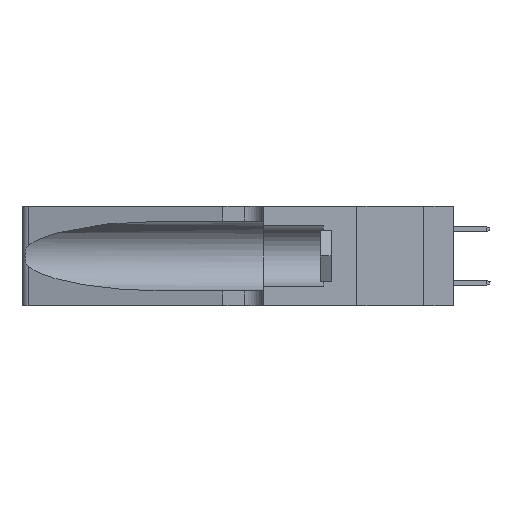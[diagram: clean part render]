
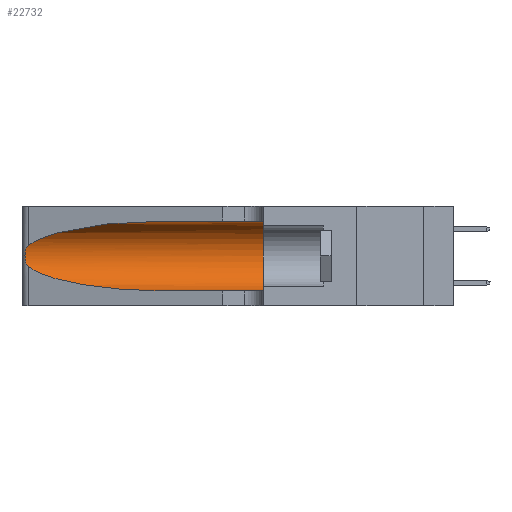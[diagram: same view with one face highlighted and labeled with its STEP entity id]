
A CAD part, left-side view. The second image highlights one B-rep face of the part: STEP entity #22732.
In plain terms, the highlighted cylindrical face has radius 3.308 mm (diameter 6.617 mm), a partial arc.
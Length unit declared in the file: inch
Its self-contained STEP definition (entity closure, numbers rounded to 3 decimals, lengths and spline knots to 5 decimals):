
#939 = VERTEX_POINT ( 'NONE', #15543 ) ;
#1526 = CARTESIAN_POINT ( 'NONE',  ( 0.2373, 1.15595, 0.08982 ) ) ;
#2543 = B_SPLINE_CURVE_WITH_KNOTS ( 'NONE', 3,
 ( #40751, #30170, #37373, #23429, #13076, #10136, #23860, #37588, #13746, #6750, #24303, #27682, #26802, #27464 ),
 .UNSPECIFIED., .F., .F.,
 ( 4, 2, 2, 2, 2, 2, 4 ),
 ( 0., 0.00027, 0.00053, 0.00107, 0.0016, 0.00187, 0.00214 ),
 .UNSPECIFIED. ) ;
#2754 = ORIENTED_EDGE ( 'NONE', *, *, #42380, .T. ) ;
#2977 = EDGE_LOOP ( 'NONE', ( #14669, #41446, #18980, #2754, #42474, #29948 ) ) ;
#4268 = CARTESIAN_POINT ( 'NONE',  ( 0.1305, 0.35, 0.31525 ) ) ;
#5178 = LINE ( 'NONE', #26124, #29187 ) ;
#5427 = CARTESIAN_POINT ( 'NONE',  ( 0.1305, 0.35, 0.185 ) ) ;
#6022 = DIRECTION ( 'NONE',  ( 0., 0., -1. ) ) ;
#6558 = EDGE_CURVE ( 'NONE', #7128, #14911, #5178, .T. ) ;
#6750 = CARTESIAN_POINT ( 'NONE',  ( 0.25856, 1.23593, 0.16098 ) ) ;
#7128 = VERTEX_POINT ( 'NONE', #16170 ) ;
#9047 = CARTESIAN_POINT ( 'NONE',  ( 0.1305, 1.61858, 0.05475 ) ) ;
#10136 = CARTESIAN_POINT ( 'NONE',  ( 0.26018, 1.23835, 0.19895 ) ) ;
#10517 = AXIS2_PLACEMENT_3D ( 'NONE', #29884, #30325, #6022 ) ;
#11136 = CARTESIAN_POINT ( 'NONE',  ( 0.25487, 1.22718, 0.22369 ) ) ;
#11793 = CARTESIAN_POINT ( 'NONE',  ( 0.18966, 0.96281, 0.31525 ) ) ;
#12193 = DIRECTION ( 'NONE',  ( 0., 1., 0. ) ) ;
#12660 = EDGE_CURVE ( 'NONE', #7128, #15549, #13015, .T. ) ;
#12906 = CIRCLE ( 'NONE', #36617, 0.13025 ) ;
#12931 = VECTOR ( 'NONE', #24326, 39.37008 ) ;
#13015 =( BOUNDED_CURVE ( )  B_SPLINE_CURVE ( 3, ( #35007, #11793, #15176, #11136 ),
 .UNSPECIFIED., .F., .F. ) 
 B_SPLINE_CURVE_WITH_KNOTS ( ( 4, 4 ),
 ( 1.5708, 2.84003 ),
 .UNSPECIFIED. ) 
 CURVE ( )  GEOMETRIC_REPRESENTATION_ITEM ( )  RATIONAL_B_SPLINE_CURVE ( ( 1., 0.87, 0.87, 1. ) ) 
 REPRESENTATION_ITEM ( '' )  );
#13076 = CARTESIAN_POINT ( 'NONE',  ( 0.25854, 1.2359, 0.20912 ) ) ;
#13659 = CARTESIAN_POINT ( 'NONE',  ( 0.25487, 1.22718, 0.22369 ) ) ;
#13746 = CARTESIAN_POINT ( 'NONE',  ( 0.26017, 1.23833, 0.17102 ) ) ;
#14669 = ORIENTED_EDGE ( 'NONE', *, *, #12660, .T. ) ;
#14911 = VERTEX_POINT ( 'NONE', #4268 ) ;
#15176 = CARTESIAN_POINT ( 'NONE',  ( 0.2373, 1.15595, 0.28018 ) ) ;
#15543 = CARTESIAN_POINT ( 'NONE',  ( 0.1305, 0.35, 0.05475 ) ) ;
#15549 = VERTEX_POINT ( 'NONE', #13659 ) ;
#16170 = CARTESIAN_POINT ( 'NONE',  ( 0.1305, 0.72297, 0.31525 ) ) ;
#18980 = ORIENTED_EDGE ( 'NONE', *, *, #43089, .T. ) ;
#20682 = CARTESIAN_POINT ( 'NONE',  ( 0.1305, 0.72297, 0.05475 ) ) ;
#20790 =( BOUNDED_CURVE ( )  B_SPLINE_CURVE ( 3, ( #38215, #1526, #21799, #25174 ),
 .UNSPECIFIED., .F., .F. ) 
 B_SPLINE_CURVE_WITH_KNOTS ( ( 4, 4 ),
 ( 3.44316, 4.71239 ),
 .UNSPECIFIED. ) 
 CURVE ( )  GEOMETRIC_REPRESENTATION_ITEM ( )  RATIONAL_B_SPLINE_CURVE ( ( 1., 0.87, 0.87, 1. ) ) 
 REPRESENTATION_ITEM ( '' )  );
#21799 = CARTESIAN_POINT ( 'NONE',  ( 0.18966, 0.96281, 0.05475 ) ) ;
#21886 = DIRECTION ( 'NONE',  ( 0., 0., 1. ) ) ;
#22732 = ADVANCED_FACE ( 'NONE', ( #43848 ), #39184, .F. ) ;
#23429 = CARTESIAN_POINT ( 'NONE',  ( 0.25787, 1.23484, 0.2124 ) ) ;
#23860 = CARTESIAN_POINT ( 'NONE',  ( 0.26075, 1.23896, 0.19203 ) ) ;
#24303 = CARTESIAN_POINT ( 'NONE',  ( 0.25789, 1.23486, 0.15765 ) ) ;
#24326 = DIRECTION ( 'NONE',  ( 0., -1., 0. ) ) ;
#25174 = CARTESIAN_POINT ( 'NONE',  ( 0.1305, 0.72297, 0.05475 ) ) ;
#25440 = VERTEX_POINT ( 'NONE', #25744 ) ;
#25744 = CARTESIAN_POINT ( 'NONE',  ( 0.25487, 1.22718, 0.14631 ) ) ;
#26124 = CARTESIAN_POINT ( 'NONE',  ( 0.1305, 1.61858, 0.31525 ) ) ;
#26802 = CARTESIAN_POINT ( 'NONE',  ( 0.25555, 1.22993, 0.14849 ) ) ;
#27230 = EDGE_CURVE ( 'NONE', #14911, #939, #12906, .T. ) ;
#27464 = CARTESIAN_POINT ( 'NONE',  ( 0.25487, 1.22718, 0.14631 ) ) ;
#27682 = CARTESIAN_POINT ( 'NONE',  ( 0.25639, 1.23186, 0.15144 ) ) ;
#29187 = VECTOR ( 'NONE', #39833, 39.37008 ) ;
#29884 = CARTESIAN_POINT ( 'NONE',  ( 0.1305, 1.61858, 0.185 ) ) ;
#29948 = ORIENTED_EDGE ( 'NONE', *, *, #6558, .F. ) ;
#30170 = CARTESIAN_POINT ( 'NONE',  ( 0.25555, 1.22994, 0.2215 ) ) ;
#30325 = DIRECTION ( 'NONE',  ( 0., -1., 0. ) ) ;
#34443 = EDGE_CURVE ( 'NONE', #15549, #25440, #2543, .T. ) ;
#34890 = VERTEX_POINT ( 'NONE', #20682 ) ;
#35007 = CARTESIAN_POINT ( 'NONE',  ( 0.1305, 0.72297, 0.31525 ) ) ;
#36617 = AXIS2_PLACEMENT_3D ( 'NONE', #5427, #12193, #21886 ) ;
#37373 = CARTESIAN_POINT ( 'NONE',  ( 0.25639, 1.23184, 0.21858 ) ) ;
#37588 = CARTESIAN_POINT ( 'NONE',  ( 0.26075, 1.23896, 0.178 ) ) ;
#38215 = CARTESIAN_POINT ( 'NONE',  ( 0.25487, 1.22718, 0.14631 ) ) ;
#39184 = CYLINDRICAL_SURFACE ( 'NONE', #10517, 0.13025 ) ;
#39833 = DIRECTION ( 'NONE',  ( 0., -1., 0. ) ) ;
#39868 = LINE ( 'NONE', #9047, #12931 ) ;
#40751 = CARTESIAN_POINT ( 'NONE',  ( 0.25487, 1.22718, 0.22369 ) ) ;
#41446 = ORIENTED_EDGE ( 'NONE', *, *, #34443, .T. ) ;
#42380 = EDGE_CURVE ( 'NONE', #34890, #939, #39868, .T. ) ;
#42474 = ORIENTED_EDGE ( 'NONE', *, *, #27230, .F. ) ;
#43089 = EDGE_CURVE ( 'NONE', #25440, #34890, #20790, .T. ) ;
#43848 = FACE_OUTER_BOUND ( 'NONE', #2977, .T. ) ;
